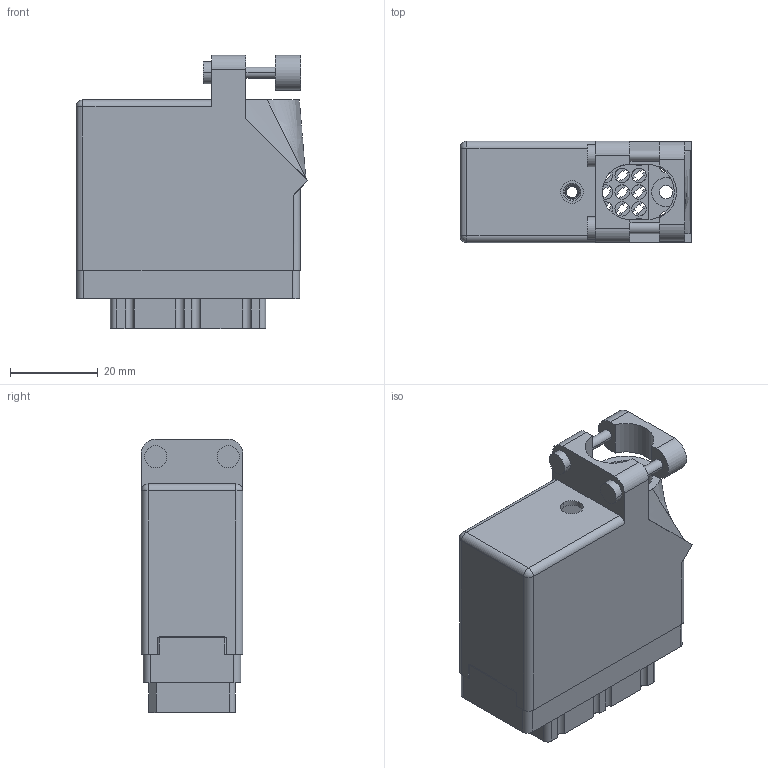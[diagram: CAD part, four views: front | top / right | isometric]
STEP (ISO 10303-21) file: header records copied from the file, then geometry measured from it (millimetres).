
FILE_DESCRIPTION (( 'STEP AP203' ), '1' );
FILE_NAME ('519-036-000-416.STEP', '2020-09-09T19:49:30', ( '' ), ( '' ), 'SwSTEP 2.0', 'SolidWorks 2020', '' );
FILE_SCHEMA (( 'CONFIG_CONTROL_DESIGN' ));
Length unit declared in the file: inch
Products named in the file (4): 516-252-035-100_516-252-035-100; 519-036-000-416; 519 Receptacle Insulator_036; 516-230-001_Plastic - 038 Top Entry
Assembly tree (3 placements, depth 2):
  519-036-000-416
    519 Receptacle Insulator_036
    516-252-035-100_516-252-035-100
    516-230-001_Plastic - 038 Top Entry
Bounding box: 52.85 x 23.11 x 62.26 mm (x, y, z)
Volume: 21888 mm3; surface area: 28477.7 mm2
Topology: 3 solids, 3 shells, 971 faces, 2809 edges, 1866 vertices
Faces by surface type: plane 659, cylinder 289, cone 12, bspline 9, sphere 2
Entity records: 34896 total; most frequent: CARTESIAN_POINT 8189, ORIENTED_EDGE 5614, DIRECTION 5398, EDGE_CURVE 2807, LINE 2044, VECTOR 2044, VERTEX_POINT 1866, AXIS2_PLACEMENT_3D 1677
